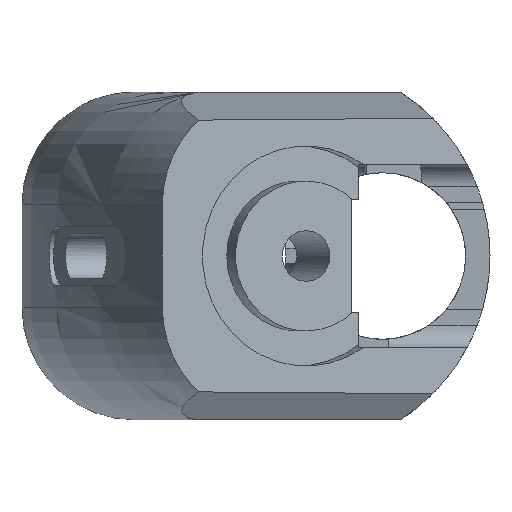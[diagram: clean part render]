
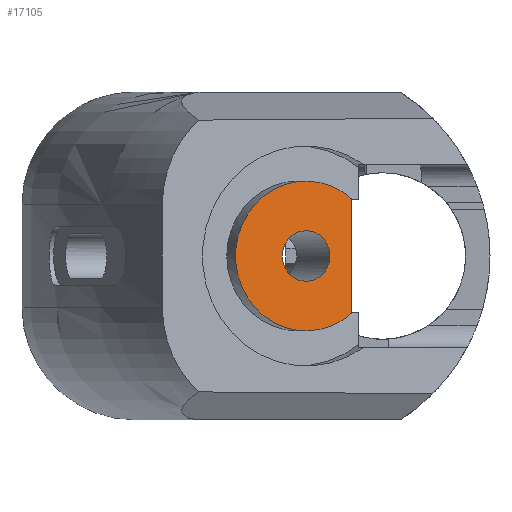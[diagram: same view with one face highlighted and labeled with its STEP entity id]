
A CAD part, left-side view. The second image highlights one B-rep face of the part: STEP entity #17105.
In plain terms, the highlighted planar face has unit normal (-0.943, -0.334, 0).
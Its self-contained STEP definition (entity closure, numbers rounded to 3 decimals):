
#3186 = PLANE('',#3187);
#3187 = AXIS2_PLACEMENT_3D('',#3188,#3189,#3190);
#3188 = CARTESIAN_POINT('',(-152.4,18.796,7.62));
#3189 = DIRECTION('',(0.,-1.,0.));
#3190 = DIRECTION('',(0.,0.,-1.));
#3235 = CYLINDRICAL_SURFACE('',#3236,3.429);
#3236 = AXIS2_PLACEMENT_3D('',#3237,#3238,#3239);
#3237 = CARTESIAN_POINT('',(-202.64,24.947,
    0.));
#3238 = DIRECTION('',(-0.943,-0.334,0.
    ));
#3239 = DIRECTION('',(0.334,-0.943,0.
    ));
#9206 = CYLINDRICAL_SURFACE('',#9207,10.16);
#9207 = AXIS2_PLACEMENT_3D('',#9208,#9209,#9210);
#9208 = CARTESIAN_POINT('',(-202.64,24.947,
    0.));
#9209 = DIRECTION('',(-0.943,-0.334,
    0.));
#9210 = DIRECTION('',(0.334,-0.943,0.)
  );
#9394 = VERTEX_POINT('',#9395);
#9395 = CARTESIAN_POINT('',(-200.461,18.796,7.62));
#9409 = PLANE('',#9410);
#9410 = AXIS2_PLACEMENT_3D('',#9411,#9412,#9413);
#9411 = CARTESIAN_POINT('',(-152.4,17.78,7.62));
#9412 = DIRECTION('',(0.,0.,-1.));
#9413 = DIRECTION('',(0.,1.,0.));
#9421 = EDGE_CURVE('',#9394,#9422,#9424,.T.);
#9422 = VERTEX_POINT('',#9423);
#9423 = CARTESIAN_POINT('',(-200.461,18.796,-7.62));
#9424 = SURFACE_CURVE('',#9425,(#9429,#9435),.PCURVE_S1.);
#9425 = LINE('',#9426,#9427);
#9426 = CARTESIAN_POINT('',(-200.461,18.796,-7.303));
#9427 = VECTOR('',#9428,1.);
#9428 = DIRECTION('',(0.,0.,-1.));
#9429 = PCURVE('',#3186,#9430);
#9430 = DEFINITIONAL_REPRESENTATION('',(#9431),#9434);
#9431 = B_SPLINE_CURVE_WITH_KNOTS('',1,(#9432,#9433),.UNSPECIFIED.,.F.,
  .F.,(2,2),(-14.923,0.318),.PIECEWISE_BEZIER_KNOTS.);
#9432 = CARTESIAN_POINT('',(0.,-48.061));
#9433 = CARTESIAN_POINT('',(15.24,-48.061));
#9434 = ( GEOMETRIC_REPRESENTATION_CONTEXT(2) 
PARAMETRIC_REPRESENTATION_CONTEXT() REPRESENTATION_CONTEXT('2D SPACE',''
  ) );
#9435 = PCURVE('',#9436,#9441);
#9436 = PLANE('',#9437);
#9437 = AXIS2_PLACEMENT_3D('',#9438,#9439,#9440);
#9438 = CARTESIAN_POINT('',(-209.55,44.45,-22.225));
#9439 = DIRECTION('',(0.943,0.334,0.)
  );
#9440 = DIRECTION('',(0.334,-0.943,0.)
  );
#9441 = DEFINITIONAL_REPRESENTATION('',(#9442),#9445);
#9442 = B_SPLINE_CURVE_WITH_KNOTS('',1,(#9443,#9444),.UNSPECIFIED.,.F.,
  .F.,(2,2),(-14.923,0.318),.PIECEWISE_BEZIER_KNOTS.);
#9443 = CARTESIAN_POINT('',(27.216,-29.845));
#9444 = CARTESIAN_POINT('',(27.216,-14.605));
#9445 = ( GEOMETRIC_REPRESENTATION_CONTEXT(2) 
PARAMETRIC_REPRESENTATION_CONTEXT() REPRESENTATION_CONTEXT('2D SPACE',''
  ) );
#9463 = PLANE('',#9464);
#9464 = AXIS2_PLACEMENT_3D('',#9465,#9466,#9467);
#9465 = CARTESIAN_POINT('',(-152.4,18.796,-7.62));
#9466 = DIRECTION('',(0.,0.,1.));
#9467 = DIRECTION('',(0.,-1.,0.));
#9561 = EDGE_CURVE('',#9562,#9562,#9564,.T.);
#9562 = VERTEX_POINT('',#9563);
#9563 = CARTESIAN_POINT('',(-201.495,21.715,
    0.));
#9564 = SURFACE_CURVE('',#9565,(#9570,#9577),.PCURVE_S1.);
#9565 = CIRCLE('',#9566,3.429);
#9566 = AXIS2_PLACEMENT_3D('',#9567,#9568,#9569);
#9567 = CARTESIAN_POINT('',(-202.64,24.947,
    0.));
#9568 = DIRECTION('',(-0.943,-0.334,0.)
  );
#9569 = DIRECTION('',(0.334,-0.943,0.
    ));
#9570 = PCURVE('',#3235,#9571);
#9571 = DEFINITIONAL_REPRESENTATION('',(#9572),#9576);
#9572 = LINE('',#9573,#9574);
#9573 = CARTESIAN_POINT('',(0.,0.));
#9574 = VECTOR('',#9575,1.);
#9575 = DIRECTION('',(1.,0.));
#9576 = ( GEOMETRIC_REPRESENTATION_CONTEXT(2) 
PARAMETRIC_REPRESENTATION_CONTEXT() REPRESENTATION_CONTEXT('2D SPACE',''
  ) );
#9577 = PCURVE('',#9436,#9578);
#9578 = DEFINITIONAL_REPRESENTATION('',(#9579),#9587);
#9579 = ( BOUNDED_CURVE() B_SPLINE_CURVE(2,(#9580,#9581,#9582,#9583,
#9584,#9585,#9586),.UNSPECIFIED.,.T.,.F.) B_SPLINE_CURVE_WITH_KNOTS((1,2
    ,2,2,2,1),(-2.094,0.,2.094,4.189,
6.283,8.378),.UNSPECIFIED.) CURVE() 
GEOMETRIC_REPRESENTATION_ITEM() RATIONAL_B_SPLINE_CURVE((1.,0.5,1.,0.5,
1.,0.5,1.)) REPRESENTATION_ITEM('') );
#9580 = CARTESIAN_POINT('',(24.12,-22.225));
#9581 = CARTESIAN_POINT('',(24.12,-28.164));
#9582 = CARTESIAN_POINT('',(18.976,-25.195));
#9583 = CARTESIAN_POINT('',(13.833,-22.225));
#9584 = CARTESIAN_POINT('',(18.976,-19.255));
#9585 = CARTESIAN_POINT('',(24.12,-16.286));
#9586 = CARTESIAN_POINT('',(24.12,-22.225));
#9587 = ( GEOMETRIC_REPRESENTATION_CONTEXT(2) 
PARAMETRIC_REPRESENTATION_CONTEXT() REPRESENTATION_CONTEXT('2D SPACE',''
  ) );
#16706 = EDGE_CURVE('',#16707,#16709,#16711,.T.);
#16707 = VERTEX_POINT('',#16708);
#16708 = CARTESIAN_POINT('',(-200.396,18.613,7.62));
#16709 = VERTEX_POINT('',#16710);
#16710 = CARTESIAN_POINT('',(-200.396,18.613,-7.62));
#16711 = SURFACE_CURVE('',#16712,(#16717,#16724),.PCURVE_S1.);
#16712 = CIRCLE('',#16713,10.16);
#16713 = AXIS2_PLACEMENT_3D('',#16714,#16715,#16716);
#16714 = CARTESIAN_POINT('',(-202.64,24.947,
    0.));
#16715 = DIRECTION('',(-0.943,-0.334,
    0.));
#16716 = DIRECTION('',(0.334,-0.943,0.)
  );
#16717 = PCURVE('',#9206,#16718);
#16718 = DEFINITIONAL_REPRESENTATION('',(#16719),#16723);
#16719 = LINE('',#16720,#16721);
#16720 = CARTESIAN_POINT('',(0.,0.));
#16721 = VECTOR('',#16722,1.);
#16722 = DIRECTION('',(1.,0.));
#16723 = ( GEOMETRIC_REPRESENTATION_CONTEXT(2) 
PARAMETRIC_REPRESENTATION_CONTEXT() REPRESENTATION_CONTEXT('2D SPACE',''
  ) );
#16724 = PCURVE('',#9436,#16725);
#16725 = DEFINITIONAL_REPRESENTATION('',(#16726),#16734);
#16726 = ( BOUNDED_CURVE() B_SPLINE_CURVE(2,(#16727,#16728,#16729,#16730
    ,#16731,#16732,#16733),.UNSPECIFIED.,.T.,.F.) 
B_SPLINE_CURVE_WITH_KNOTS((1,2,2,2,2,1),(-2.094,0.,
    2.094,4.189,6.283,8.378),
.UNSPECIFIED.) CURVE() GEOMETRIC_REPRESENTATION_ITEM() 
RATIONAL_B_SPLINE_CURVE((1.,0.5,1.,0.5,1.,0.5,1.)) REPRESENTATION_ITEM(
  '') );
#16727 = CARTESIAN_POINT('',(30.851,-22.225));
#16728 = CARTESIAN_POINT('',(30.851,-39.823));
#16729 = CARTESIAN_POINT('',(15.611,-31.024));
#16730 = CARTESIAN_POINT('',(0.371,-22.225));
#16731 = CARTESIAN_POINT('',(15.611,-13.426));
#16732 = CARTESIAN_POINT('',(30.851,-4.627));
#16733 = CARTESIAN_POINT('',(30.851,-22.225));
#16734 = ( GEOMETRIC_REPRESENTATION_CONTEXT(2) 
PARAMETRIC_REPRESENTATION_CONTEXT() REPRESENTATION_CONTEXT('2D SPACE',''
  ) );
#17087 = EDGE_CURVE('',#9422,#16709,#17088,.T.);
#17088 = SURFACE_CURVE('',#17089,(#17093,#17099),.PCURVE_S1.);
#17089 = LINE('',#17090,#17091);
#17090 = CARTESIAN_POINT('',(-202.326,24.059,-7.62));
#17091 = VECTOR('',#17092,1.);
#17092 = DIRECTION('',(0.334,-0.943,0.
    ));
#17093 = PCURVE('',#9463,#17094);
#17094 = DEFINITIONAL_REPRESENTATION('',(#17095),#17098);
#17095 = B_SPLINE_CURVE_WITH_KNOTS('',1,(#17096,#17097),.UNSPECIFIED.,
  .F.,.F.,(2,2),(5.583,6.661),
  .PIECEWISE_BEZIER_KNOTS.);
#17096 = CARTESIAN_POINT('',(0.,-48.061));
#17097 = CARTESIAN_POINT('',(1.016,-47.701));
#17098 = ( GEOMETRIC_REPRESENTATION_CONTEXT(2) 
PARAMETRIC_REPRESENTATION_CONTEXT() REPRESENTATION_CONTEXT('2D SPACE',''
  ) );
#17099 = PCURVE('',#9436,#17100);
#17100 = DEFINITIONAL_REPRESENTATION('',(#17101),#17104);
#17101 = B_SPLINE_CURVE_WITH_KNOTS('',1,(#17102,#17103),.UNSPECIFIED.,
  .F.,.F.,(2,2),(5.583,6.661),
  .PIECEWISE_BEZIER_KNOTS.);
#17102 = CARTESIAN_POINT('',(27.216,-14.605));
#17103 = CARTESIAN_POINT('',(28.294,-14.605));
#17104 = ( GEOMETRIC_REPRESENTATION_CONTEXT(2) 
PARAMETRIC_REPRESENTATION_CONTEXT() REPRESENTATION_CONTEXT('2D SPACE',''
  ) );
#17105 = ADVANCED_FACE('',(#17106,#17130),#9436,.F.);
#17106 = FACE_BOUND('',#17107,.F.);
#17107 = EDGE_LOOP('',(#17108,#17109,#17110,#17129));
#17108 = ORIENTED_EDGE('',*,*,#17087,.T.);
#17109 = ORIENTED_EDGE('',*,*,#16706,.F.);
#17110 = ORIENTED_EDGE('',*,*,#17111,.T.);
#17111 = EDGE_CURVE('',#16707,#9394,#17112,.T.);
#17112 = SURFACE_CURVE('',#17113,(#17117,#17123),.PCURVE_S1.);
#17113 = LINE('',#17114,#17115);
#17114 = CARTESIAN_POINT('',(-202.166,23.607,7.62));
#17115 = VECTOR('',#17116,1.);
#17116 = DIRECTION('',(-0.334,0.943,
    0.));
#17117 = PCURVE('',#9436,#17118);
#17118 = DEFINITIONAL_REPRESENTATION('',(#17119),#17122);
#17119 = B_SPLINE_CURVE_WITH_KNOTS('',1,(#17120,#17121),.UNSPECIFIED.,
  .F.,.F.,(2,2),(-6.182,-5.104),
  .PIECEWISE_BEZIER_KNOTS.);
#17120 = CARTESIAN_POINT('',(28.294,-29.845));
#17121 = CARTESIAN_POINT('',(27.216,-29.845));
#17122 = ( GEOMETRIC_REPRESENTATION_CONTEXT(2) 
PARAMETRIC_REPRESENTATION_CONTEXT() REPRESENTATION_CONTEXT('2D SPACE',''
  ) );
#17123 = PCURVE('',#9409,#17124);
#17124 = DEFINITIONAL_REPRESENTATION('',(#17125),#17128);
#17125 = B_SPLINE_CURVE_WITH_KNOTS('',1,(#17126,#17127),.UNSPECIFIED.,
  .F.,.F.,(2,2),(-6.182,-5.104),
  .PIECEWISE_BEZIER_KNOTS.);
#17126 = CARTESIAN_POINT('',(0.,-47.701));
#17127 = CARTESIAN_POINT('',(1.016,-48.061));
#17128 = ( GEOMETRIC_REPRESENTATION_CONTEXT(2) 
PARAMETRIC_REPRESENTATION_CONTEXT() REPRESENTATION_CONTEXT('2D SPACE',''
  ) );
#17129 = ORIENTED_EDGE('',*,*,#9421,.T.);
#17130 = FACE_BOUND('',#17131,.F.);
#17131 = EDGE_LOOP('',(#17132));
#17132 = ORIENTED_EDGE('',*,*,#9561,.T.);
